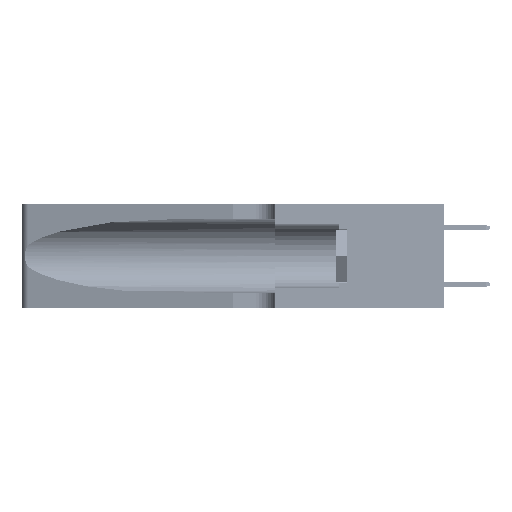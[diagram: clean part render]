
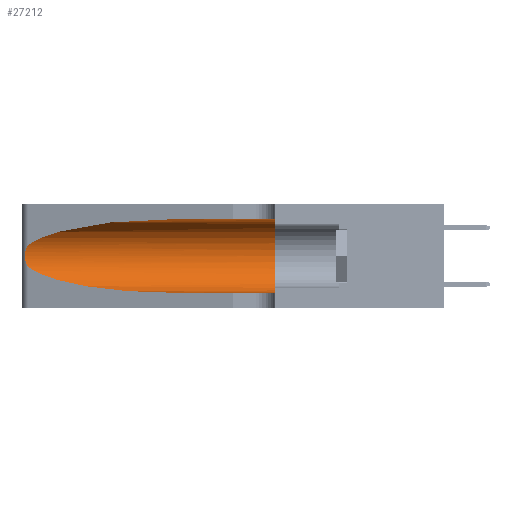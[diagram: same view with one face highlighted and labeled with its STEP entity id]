
A CAD part, left-side view. The second image highlights one B-rep face of the part: STEP entity #27212.
In plain terms, the highlighted cylindrical face has radius 3.308 mm (diameter 6.617 mm), a partial arc.
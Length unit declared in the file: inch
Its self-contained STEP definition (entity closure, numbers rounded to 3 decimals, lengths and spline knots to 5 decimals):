
#641 = CARTESIAN_POINT ( 'NONE',  ( 0.1305, 0.35, 0.05475 ) ) ;
#748 = FACE_OUTER_BOUND ( 'NONE', #13470, .T. ) ;
#788 = AXIS2_PLACEMENT_3D ( 'NONE', #28694, #1450, #32400 ) ;
#1450 = DIRECTION ( 'NONE',  ( 0., -1., 0. ) ) ;
#1568 = CARTESIAN_POINT ( 'NONE',  ( 0.25487, 1.22718, 0.22369 ) ) ;
#2809 = EDGE_CURVE ( 'NONE', #4309, #18894, #46803, .T. ) ;
#4309 = VERTEX_POINT ( 'NONE', #35728 ) ;
#4674 = VECTOR ( 'NONE', #32989, 39.37008 ) ;
#4986 = EDGE_CURVE ( 'NONE', #13845, #27530, #38162, .T. ) ;
#5210 = CARTESIAN_POINT ( 'NONE',  ( 0.1305, 0.35, 0.31525 ) ) ;
#5497 = CARTESIAN_POINT ( 'NONE',  ( 0.25854, 1.2359, 0.20912 ) ) ;
#5939 = CARTESIAN_POINT ( 'NONE',  ( 0.1305, 0.72297, 0.05475 ) ) ;
#6542 = CARTESIAN_POINT ( 'NONE',  ( 0.1305, 0.72297, 0.31525 ) ) ;
#8751 = CYLINDRICAL_SURFACE ( 'NONE', #788, 0.13025 ) ;
#9110 = CARTESIAN_POINT ( 'NONE',  ( 0.1305, 0.35, 0.185 ) ) ;
#9433 = CARTESIAN_POINT ( 'NONE',  ( 0.26075, 1.23896, 0.19203 ) ) ;
#9696 = CARTESIAN_POINT ( 'NONE',  ( 0.25487, 1.22718, 0.14631 ) ) ;
#9897 = VERTEX_POINT ( 'NONE', #6542 ) ;
#10425 = EDGE_CURVE ( 'NONE', #9897, #37261, #16235, .T. ) ;
#11176 =( BOUNDED_CURVE ( )  B_SPLINE_CURVE ( 3, ( #28432, #32314, #12956, #39992 ),
 .UNSPECIFIED., .F., .T. ) 
 B_SPLINE_CURVE_WITH_KNOTS ( ( 4, 4 ),
 ( 1.5708, 2.84003 ),
 .UNSPECIFIED. ) 
 CURVE ( )  GEOMETRIC_REPRESENTATION_ITEM ( )  RATIONAL_B_SPLINE_CURVE ( ( 1., 0.87, 0.87, 1. ) ) 
 REPRESENTATION_ITEM ( '' )  );
#12956 = CARTESIAN_POINT ( 'NONE',  ( 0.2373, 1.15595, 0.28018 ) ) ;
#13016 = DIRECTION ( 'NONE',  ( 0., 0., 1. ) ) ;
#13168 = CARTESIAN_POINT ( 'NONE',  ( 0.25639, 1.23184, 0.21858 ) ) ;
#13340 = CARTESIAN_POINT ( 'NONE',  ( 0.26017, 1.23833, 0.17102 ) ) ;
#13470 = EDGE_LOOP ( 'NONE', ( #29727, #47817, #22751, #18000, #17060, #41855 ) ) ;
#13527 = EDGE_CURVE ( 'NONE', #37261, #18894, #35280, .T. ) ;
#13845 = VERTEX_POINT ( 'NONE', #46229 ) ;
#16235 = LINE ( 'NONE', #29121, #4674 ) ;
#16504 =( BOUNDED_CURVE ( )  B_SPLINE_CURVE ( 3, ( #9696, #32951, #29244, #5939 ),
 .UNSPECIFIED., .F., .T. ) 
 B_SPLINE_CURVE_WITH_KNOTS ( ( 4, 4 ),
 ( 3.44316, 4.71239 ),
 .UNSPECIFIED. ) 
 CURVE ( )  GEOMETRIC_REPRESENTATION_ITEM ( )  RATIONAL_B_SPLINE_CURVE ( ( 1., 0.87, 0.87, 1. ) ) 
 REPRESENTATION_ITEM ( '' )  );
#17060 = ORIENTED_EDGE ( 'NONE', *, *, #13527, .F. ) ;
#17231 = CARTESIAN_POINT ( 'NONE',  ( 0.25789, 1.23486, 0.15765 ) ) ;
#18000 = ORIENTED_EDGE ( 'NONE', *, *, #2809, .T. ) ;
#18894 = VERTEX_POINT ( 'NONE', #641 ) ;
#18991 = EDGE_CURVE ( 'NONE', #9897, #13845, #11176, .T. ) ;
#21155 = CARTESIAN_POINT ( 'NONE',  ( 0.25555, 1.22993, 0.14849 ) ) ;
#22751 = ORIENTED_EDGE ( 'NONE', *, *, #42844, .T. ) ;
#24946 = AXIS2_PLACEMENT_3D ( 'NONE', #9110, #36205, #13016 ) ;
#27212 = ADVANCED_FACE ( 'NONE', ( #748 ), #8751, .F. ) ;
#27530 = VERTEX_POINT ( 'NONE', #34190 ) ;
#28432 = CARTESIAN_POINT ( 'NONE',  ( 0.1305, 0.72297, 0.31525 ) ) ;
#28694 = CARTESIAN_POINT ( 'NONE',  ( 0.1305, 1.61858, 0.185 ) ) ;
#28810 = CARTESIAN_POINT ( 'NONE',  ( 0.25787, 1.23484, 0.2124 ) ) ;
#29121 = CARTESIAN_POINT ( 'NONE',  ( 0.1305, 1.61858, 0.31525 ) ) ;
#29244 = CARTESIAN_POINT ( 'NONE',  ( 0.18966, 0.96281, 0.05475 ) ) ;
#29727 = ORIENTED_EDGE ( 'NONE', *, *, #18991, .T. ) ;
#32314 = CARTESIAN_POINT ( 'NONE',  ( 0.18966, 0.96281, 0.31525 ) ) ;
#32400 = DIRECTION ( 'NONE',  ( 0., 0., -1. ) ) ;
#32677 = CARTESIAN_POINT ( 'NONE',  ( 0.26018, 1.23835, 0.19895 ) ) ;
#32951 = CARTESIAN_POINT ( 'NONE',  ( 0.2373, 1.15595, 0.08982 ) ) ;
#32989 = DIRECTION ( 'NONE',  ( 0., -1., 0. ) ) ;
#34190 = CARTESIAN_POINT ( 'NONE',  ( 0.25487, 1.22718, 0.14631 ) ) ;
#35280 = CIRCLE ( 'NONE', #24946, 0.13025 ) ;
#35728 = CARTESIAN_POINT ( 'NONE',  ( 0.1305, 0.72297, 0.05475 ) ) ;
#36205 = DIRECTION ( 'NONE',  ( 0., 1., 0. ) ) ;
#36517 = CARTESIAN_POINT ( 'NONE',  ( 0.26075, 1.23896, 0.178 ) ) ;
#36608 = VECTOR ( 'NONE', #42706, 39.37008 ) ;
#37261 = VERTEX_POINT ( 'NONE', #5210 ) ;
#38162 = B_SPLINE_CURVE_WITH_KNOTS ( 'NONE', 3,
 ( #1568, #44077, #13168, #28810, #5497, #32677, #9433, #36517, #13340, #40372, #17231, #44239, #21155, #48099 ),
 .UNSPECIFIED., .F., .F.,
 ( 4, 2, 2, 2, 2, 2, 4 ),
 ( 0., 0.00027, 0.00053, 0.00107, 0.0016, 0.00187, 0.00214 ),
 .UNSPECIFIED. ) ;
#39992 = CARTESIAN_POINT ( 'NONE',  ( 0.25487, 1.22718, 0.22369 ) ) ;
#40372 = CARTESIAN_POINT ( 'NONE',  ( 0.25856, 1.23593, 0.16098 ) ) ;
#41855 = ORIENTED_EDGE ( 'NONE', *, *, #10425, .F. ) ;
#42548 = CARTESIAN_POINT ( 'NONE',  ( 0.1305, 1.61858, 0.05475 ) ) ;
#42706 = DIRECTION ( 'NONE',  ( 0., -1., 0. ) ) ;
#42844 = EDGE_CURVE ( 'NONE', #27530, #4309, #16504, .T. ) ;
#44077 = CARTESIAN_POINT ( 'NONE',  ( 0.25555, 1.22994, 0.2215 ) ) ;
#44239 = CARTESIAN_POINT ( 'NONE',  ( 0.25639, 1.23186, 0.15144 ) ) ;
#46229 = CARTESIAN_POINT ( 'NONE',  ( 0.25487, 1.22718, 0.22369 ) ) ;
#46803 = LINE ( 'NONE', #42548, #36608 ) ;
#47817 = ORIENTED_EDGE ( 'NONE', *, *, #4986, .T. ) ;
#48099 = CARTESIAN_POINT ( 'NONE',  ( 0.25487, 1.22718, 0.14631 ) ) ;
